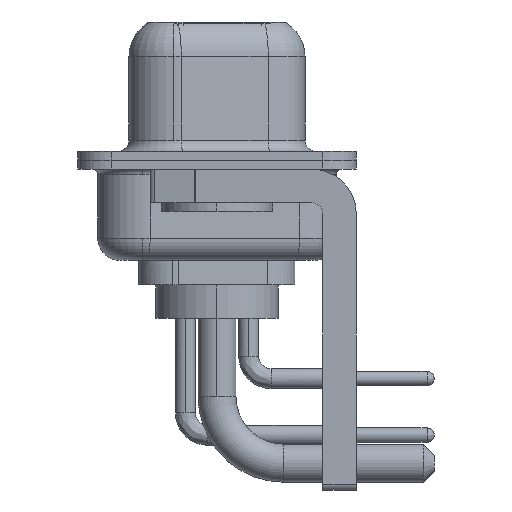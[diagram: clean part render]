
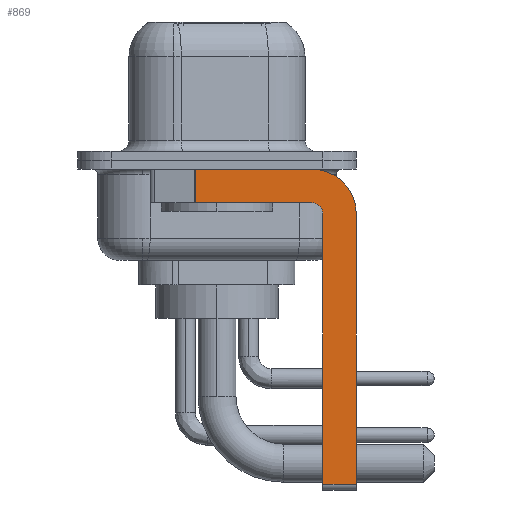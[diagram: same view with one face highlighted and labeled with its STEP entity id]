
A CAD part, left-side view. The second image highlights one B-rep face of the part: STEP entity #869.
In plain terms, the highlighted planar face has unit normal (-1, 0, 0).
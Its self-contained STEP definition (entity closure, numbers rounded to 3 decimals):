
#159 = CARTESIAN_POINT ( 'NONE',  ( -2.9, -4.25, -14.55 ) ) ;
#492 = VECTOR ( 'NONE', #2682, 1000. ) ;
#531 = CARTESIAN_POINT ( 'NONE',  ( -2.9, -4.25, -2.4 ) ) ;
#869 = ADVANCED_FACE ( 'NONE', ( #1199 ), #14515, .F. ) ;
#1136 = DIRECTION ( 'NONE',  ( 0., 0., 1. ) ) ;
#1199 = FACE_OUTER_BOUND ( 'NONE', #11260, .T. ) ;
#1235 = ORIENTED_EDGE ( 'NONE', *, *, #10247, .T. ) ;
#1448 = ORIENTED_EDGE ( 'NONE', *, *, #3057, .F. ) ;
#1859 = ORIENTED_EDGE ( 'NONE', *, *, #15112, .F. ) ;
#2103 = VECTOR ( 'NONE', #7113, 1000. ) ;
#2292 = VERTEX_POINT ( 'NONE', #13590 ) ;
#2620 = CARTESIAN_POINT ( 'NONE',  ( -2.9, -6.25, -14.55 ) ) ;
#2682 = DIRECTION ( 'NONE',  ( 0., 1., 0. ) ) ;
#3057 = EDGE_CURVE ( 'NONE', #10892, #12942, #14983, .T. ) ;
#3859 = ORIENTED_EDGE ( 'NONE', *, *, #9625, .F. ) ;
#3947 = CARTESIAN_POINT ( 'NONE',  ( -2.9, 0.978, -0.4 ) ) ;
#4684 = EDGE_CURVE ( 'NONE', #13993, #6049, #8610, .T. ) ;
#4757 = VECTOR ( 'NONE', #14752, 1000. ) ;
#4961 = CARTESIAN_POINT ( 'NONE',  ( -2.9, -4.25, -2.4 ) ) ;
#5031 = CARTESIAN_POINT ( 'NONE',  ( -2.9, 0.978, -1.9 ) ) ;
#5502 = CARTESIAN_POINT ( 'NONE',  ( -2.9, -4.75, -14.55 ) ) ;
#5845 = DIRECTION ( 'NONE',  ( 0., 0., 1. ) ) ;
#6049 = VERTEX_POINT ( 'NONE', #7648 ) ;
#6321 = CARTESIAN_POINT ( 'NONE',  ( -2.9, 0.978, -1.9 ) ) ;
#6444 = VECTOR ( 'NONE', #14109, 1000. ) ;
#6650 = VERTEX_POINT ( 'NONE', #2620 ) ;
#7113 = DIRECTION ( 'NONE',  ( 0., -1., 0. ) ) ;
#7648 = CARTESIAN_POINT ( 'NONE',  ( -2.9, -4.75, -2.4 ) ) ;
#7717 = DIRECTION ( 'NONE',  ( 0., 0., -1. ) ) ;
#8025 = EDGE_CURVE ( 'NONE', #15845, #15098, #9309, .T. ) ;
#8231 = CIRCLE ( 'NONE', #17363, 0.5 ) ;
#8308 = CARTESIAN_POINT ( 'NONE',  ( -2.9, -4.25, -1.9 ) ) ;
#8548 = VECTOR ( 'NONE', #10485, 1000. ) ;
#8610 = LINE ( 'NONE', #15501, #11274 ) ;
#8732 = ORIENTED_EDGE ( 'NONE', *, *, #12825, .F. ) ;
#9264 = AXIS2_PLACEMENT_3D ( 'NONE', #4961, #10407, #12008 ) ;
#9283 = CARTESIAN_POINT ( 'NONE',  ( -2.9, -6.25, -2.4 ) ) ;
#9309 = LINE ( 'NONE', #5031, #8548 ) ;
#9625 = EDGE_CURVE ( 'NONE', #2292, #15098, #13578, .T. ) ;
#9682 = CARTESIAN_POINT ( 'NONE',  ( -2.9, -4.25, -0.4 ) ) ;
#9725 = CARTESIAN_POINT ( 'NONE',  ( -2.9, 3., -0.4 ) ) ;
#9797 = EDGE_CURVE ( 'NONE', #15845, #10892, #9903, .T. ) ;
#9903 = LINE ( 'NONE', #9725, #6444 ) ;
#10247 = EDGE_CURVE ( 'NONE', #13993, #6650, #13905, .T. ) ;
#10389 = ORIENTED_EDGE ( 'NONE', *, *, #8025, .T. ) ;
#10407 = DIRECTION ( 'NONE',  ( 1., 0., 0. ) ) ;
#10485 = DIRECTION ( 'NONE',  ( 0., 0., -1. ) ) ;
#10637 = LINE ( 'NONE', #9283, #4757 ) ;
#10892 = VERTEX_POINT ( 'NONE', #9682 ) ;
#11260 = EDGE_LOOP ( 'NONE', ( #13528, #10389, #3859, #1859, #12877, #1235, #8732, #1448 ) ) ;
#11274 = VECTOR ( 'NONE', #5845, 1000. ) ;
#11493 = DIRECTION ( 'NONE',  ( -1., 0., 0. ) ) ;
#12008 = DIRECTION ( 'NONE',  ( 0., 0., -1. ) ) ;
#12085 = CARTESIAN_POINT ( 'NONE',  ( -2.9, -4.25, -2.4 ) ) ;
#12825 = EDGE_CURVE ( 'NONE', #12942, #6650, #10637, .T. ) ;
#12877 = ORIENTED_EDGE ( 'NONE', *, *, #4684, .F. ) ;
#12942 = VERTEX_POINT ( 'NONE', #13932 ) ;
#13528 = ORIENTED_EDGE ( 'NONE', *, *, #9797, .F. ) ;
#13578 = LINE ( 'NONE', #8308, #492 ) ;
#13590 = CARTESIAN_POINT ( 'NONE',  ( -2.9, -4.25, -1.9 ) ) ;
#13905 = LINE ( 'NONE', #159, #2103 ) ;
#13932 = CARTESIAN_POINT ( 'NONE',  ( -2.9, -6.25, -2.4 ) ) ;
#13993 = VERTEX_POINT ( 'NONE', #5502 ) ;
#14109 = DIRECTION ( 'NONE',  ( 0., -1., 0. ) ) ;
#14515 = PLANE ( 'NONE',  #15506 ) ;
#14602 = DIRECTION ( 'NONE',  ( 1., 0., 0. ) ) ;
#14752 = DIRECTION ( 'NONE',  ( 0., 0., -1. ) ) ;
#14983 = CIRCLE ( 'NONE', #9264, 2. ) ;
#15098 = VERTEX_POINT ( 'NONE', #6321 ) ;
#15112 = EDGE_CURVE ( 'NONE', #6049, #2292, #8231, .T. ) ;
#15501 = CARTESIAN_POINT ( 'NONE',  ( -2.9, -4.75, -14.8 ) ) ;
#15506 = AXIS2_PLACEMENT_3D ( 'NONE', #12085, #14602, #7717 ) ;
#15845 = VERTEX_POINT ( 'NONE', #3947 ) ;
#17363 = AXIS2_PLACEMENT_3D ( 'NONE', #531, #11493, #1136 ) ;
